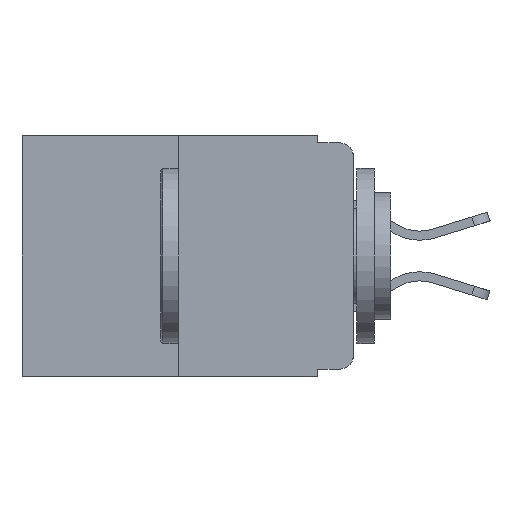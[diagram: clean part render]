
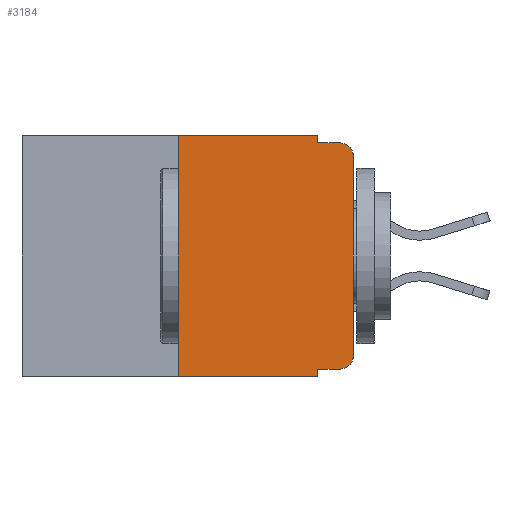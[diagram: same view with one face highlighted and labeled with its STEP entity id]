
A CAD part, left-side view. The second image highlights one B-rep face of the part: STEP entity #3184.
In plain terms, the highlighted planar face has unit normal (-1, 0, 0).
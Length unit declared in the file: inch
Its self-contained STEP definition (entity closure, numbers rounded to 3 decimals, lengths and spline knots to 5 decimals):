
#67 = DIRECTION ( 'NONE',  ( 0., 0., -1. ) ) ;
#457 = VERTEX_POINT ( 'NONE', #7798 ) ;
#1313 = EDGE_CURVE ( 'NONE', #17587, #4286, #20659, .T. ) ;
#1401 = CARTESIAN_POINT ( 'NONE',  ( 0., 0., -0.03 ) ) ;
#1465 = ORIENTED_EDGE ( 'NONE', *, *, #23398, .F. ) ;
#2089 = DIRECTION ( 'NONE',  ( 0., 0., -1. ) ) ;
#2410 = ORIENTED_EDGE ( 'NONE', *, *, #1313, .T. ) ;
#2650 = EDGE_CURVE ( 'NONE', #17587, #14835, #7255, .T. ) ;
#2702 = VERTEX_POINT ( 'NONE', #1401 ) ;
#3085 = LINE ( 'NONE', #13227, #7757 ) ;
#3119 = CARTESIAN_POINT ( 'NONE',  ( 0., 0.25, 0. ) ) ;
#3184 = ADVANCED_FACE ( 'NONE', ( #11203 ), #3719, .F. ) ;
#3487 = CARTESIAN_POINT ( 'NONE',  ( 0., 0.02, -0.313 ) ) ;
#3719 = PLANE ( 'NONE',  #8322 ) ;
#3802 = CARTESIAN_POINT ( 'NONE',  ( 0., 0.25, 0. ) ) ;
#4165 = CARTESIAN_POINT ( 'NONE',  ( 0., 0.051, -0.333 ) ) ;
#4286 = VERTEX_POINT ( 'NONE', #6695 ) ;
#4477 = VECTOR ( 'NONE', #67, 39.37008 ) ;
#4584 = ORIENTED_EDGE ( 'NONE', *, *, #11923, .F. ) ;
#5236 = LINE ( 'NONE', #14982, #20054 ) ;
#5489 = DIRECTION ( 'NONE',  ( 0., 0., -1. ) ) ;
#5737 = VECTOR ( 'NONE', #20582, 39.37008 ) ;
#5794 = DIRECTION ( 'NONE',  ( -1., 0., 0. ) ) ;
#5917 = DIRECTION ( 'NONE',  ( 1., 0., 0. ) ) ;
#6173 = EDGE_CURVE ( 'NONE', #2702, #13656, #19142, .T. ) ;
#6600 = CARTESIAN_POINT ( 'NONE',  ( 0., 0.473, 0. ) ) ;
#6695 = CARTESIAN_POINT ( 'NONE',  ( 0., 0.02, -0.333 ) ) ;
#6955 = CARTESIAN_POINT ( 'NONE',  ( 0., 0.02, -0.01 ) ) ;
#7255 = LINE ( 'NONE', #24421, #12434 ) ;
#7455 = DIRECTION ( 'NONE',  ( 0., -1., 0. ) ) ;
#7520 = CIRCLE ( 'NONE', #20306, 0.02 ) ;
#7700 = CARTESIAN_POINT ( 'NONE',  ( 0., 0.051, 0. ) ) ;
#7757 = VECTOR ( 'NONE', #22687, 39.37008 ) ;
#7798 = CARTESIAN_POINT ( 'NONE',  ( 0., 0.25, -0.343 ) ) ;
#8322 = AXIS2_PLACEMENT_3D ( 'NONE', #6600, #5917, #16216 ) ;
#8595 = ORIENTED_EDGE ( 'NONE', *, *, #16857, .F. ) ;
#8773 = CARTESIAN_POINT ( 'NONE',  ( 0., 0.051, -0.01 ) ) ;
#8796 = LINE ( 'NONE', #12284, #15200 ) ;
#9692 = CARTESIAN_POINT ( 'NONE',  ( 0., 0.051, -0.333 ) ) ;
#10733 = ORIENTED_EDGE ( 'NONE', *, *, #6173, .T. ) ;
#11203 = FACE_OUTER_BOUND ( 'NONE', #12223, .T. ) ;
#11923 = EDGE_CURVE ( 'NONE', #457, #23511, #17293, .T. ) ;
#12223 = EDGE_LOOP ( 'NONE', ( #14689, #10733, #1465, #17677, #8595, #4584, #20637, #16779, #2410, #14714 ) ) ;
#12284 = CARTESIAN_POINT ( 'NONE',  ( 0., 0., 0. ) ) ;
#12434 = VECTOR ( 'NONE', #2089, 39.37008 ) ;
#12746 = VERTEX_POINT ( 'NONE', #7700 ) ;
#13008 = VECTOR ( 'NONE', #7455, 39.37008 ) ;
#13227 = CARTESIAN_POINT ( 'NONE',  ( 0., 0.473, 0. ) ) ;
#13616 = LINE ( 'NONE', #17090, #13008 ) ;
#13656 = VERTEX_POINT ( 'NONE', #6955 ) ;
#14421 = VERTEX_POINT ( 'NONE', #16990 ) ;
#14689 = ORIENTED_EDGE ( 'NONE', *, *, #21188, .T. ) ;
#14714 = ORIENTED_EDGE ( 'NONE', *, *, #22608, .T. ) ;
#14755 = AXIS2_PLACEMENT_3D ( 'NONE', #17422, #5794, #19330 ) ;
#14835 = VERTEX_POINT ( 'NONE', #24065 ) ;
#14890 = LINE ( 'NONE', #15771, #4477 ) ;
#14982 = CARTESIAN_POINT ( 'NONE',  ( 0., 0.473, -0.343 ) ) ;
#15200 = VECTOR ( 'NONE', #23674, 39.37008 ) ;
#15624 = VECTOR ( 'NONE', #22407, 39.37008 ) ;
#15771 = CARTESIAN_POINT ( 'NONE',  ( 0., 0.051, 0. ) ) ;
#16216 = DIRECTION ( 'NONE',  ( 0., 0., -1. ) ) ;
#16779 = ORIENTED_EDGE ( 'NONE', *, *, #2650, .F. ) ;
#16857 = EDGE_CURVE ( 'NONE', #23511, #12746, #3085, .T. ) ;
#16874 = DIRECTION ( 'NONE',  ( 0., -1., 0. ) ) ;
#16990 = CARTESIAN_POINT ( 'NONE',  ( 0., 0., -0.313 ) ) ;
#17090 = CARTESIAN_POINT ( 'NONE',  ( 0., 0.051, -0.01 ) ) ;
#17115 = DIRECTION ( 'NONE',  ( -1., 0., 0. ) ) ;
#17293 = LINE ( 'NONE', #3119, #5737 ) ;
#17417 = EDGE_CURVE ( 'NONE', #457, #14835, #5236, .T. ) ;
#17422 = CARTESIAN_POINT ( 'NONE',  ( 0., 0.02, -0.03 ) ) ;
#17587 = VERTEX_POINT ( 'NONE', #9692 ) ;
#17677 = ORIENTED_EDGE ( 'NONE', *, *, #19598, .F. ) ;
#19142 = CIRCLE ( 'NONE', #14755, 0.02 ) ;
#19330 = DIRECTION ( 'NONE',  ( 0., 0., -1. ) ) ;
#19598 = EDGE_CURVE ( 'NONE', #12746, #23886, #14890, .T. ) ;
#20054 = VECTOR ( 'NONE', #16874, 39.37008 ) ;
#20306 = AXIS2_PLACEMENT_3D ( 'NONE', #3487, #17115, #5489 ) ;
#20582 = DIRECTION ( 'NONE',  ( 0., 0., 1. ) ) ;
#20637 = ORIENTED_EDGE ( 'NONE', *, *, #17417, .T. ) ;
#20659 = LINE ( 'NONE', #4165, #15624 ) ;
#21188 = EDGE_CURVE ( 'NONE', #14421, #2702, #8796, .T. ) ;
#22407 = DIRECTION ( 'NONE',  ( 0., -1., 0. ) ) ;
#22608 = EDGE_CURVE ( 'NONE', #4286, #14421, #7520, .T. ) ;
#22687 = DIRECTION ( 'NONE',  ( 0., -1., 0. ) ) ;
#23398 = EDGE_CURVE ( 'NONE', #23886, #13656, #13616, .T. ) ;
#23511 = VERTEX_POINT ( 'NONE', #3802 ) ;
#23674 = DIRECTION ( 'NONE',  ( 0., 0., 1. ) ) ;
#23886 = VERTEX_POINT ( 'NONE', #8773 ) ;
#24065 = CARTESIAN_POINT ( 'NONE',  ( 0., 0.051, -0.343 ) ) ;
#24421 = CARTESIAN_POINT ( 'NONE',  ( 0., 0.051, 0. ) ) ;
